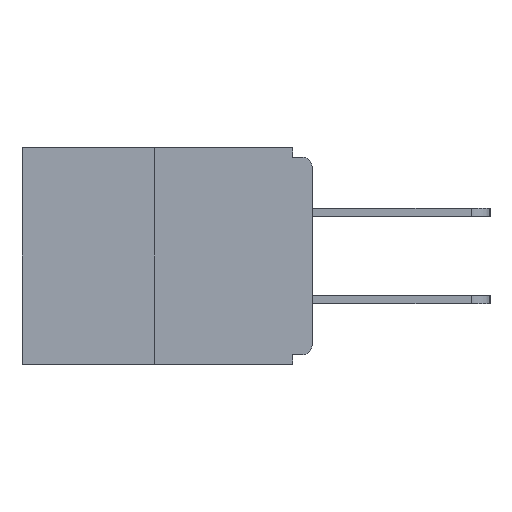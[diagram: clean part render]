
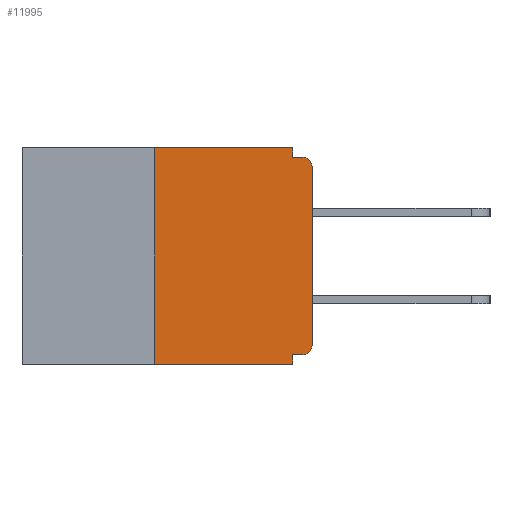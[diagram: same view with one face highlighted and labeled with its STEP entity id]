
A CAD part, left-side view. The second image highlights one B-rep face of the part: STEP entity #11995.
In plain terms, the highlighted planar face has unit normal (-1, 0, 0).
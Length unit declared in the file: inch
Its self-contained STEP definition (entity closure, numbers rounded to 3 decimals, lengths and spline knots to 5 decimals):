
#1243 = CARTESIAN_POINT ( 'NONE',  ( 0., 0.031, 0. ) ) ;
#1306 = CARTESIAN_POINT ( 'NONE',  ( 0., 0.015, -0.313 ) ) ;
#1724 = LINE ( 'NONE', #29578, #30175 ) ;
#1776 = LINE ( 'NONE', #13840, #30394 ) ;
#2646 = AXIS2_PLACEMENT_3D ( 'NONE', #10609, #20037, #5965 ) ;
#2881 = ORIENTED_EDGE ( 'NONE', *, *, #13400, .T. ) ;
#2993 = EDGE_CURVE ( 'NONE', #8689, #3377, #6218, .T. ) ;
#3151 = CIRCLE ( 'NONE', #2646, 0.015 ) ;
#3377 = VERTEX_POINT ( 'NONE', #12689 ) ;
#3730 = LINE ( 'NONE', #1243, #15689 ) ;
#3793 = DIRECTION ( 'NONE',  ( -1., 0., 0. ) ) ;
#4022 = DIRECTION ( 'NONE',  ( 0., 0., -1. ) ) ;
#4214 = VERTEX_POINT ( 'NONE', #24822 ) ;
#4319 = LINE ( 'NONE', #18544, #5563 ) ;
#4607 = VERTEX_POINT ( 'NONE', #19976 ) ;
#5035 = VECTOR ( 'NONE', #22142, 39.37008 ) ;
#5097 = DIRECTION ( 'NONE',  ( 0., 0., 1. ) ) ;
#5397 = VERTEX_POINT ( 'NONE', #9967 ) ;
#5511 = VERTEX_POINT ( 'NONE', #10764 ) ;
#5563 = VECTOR ( 'NONE', #29996, 39.37008 ) ;
#5786 = CARTESIAN_POINT ( 'NONE',  ( 0., 0.46, 0. ) ) ;
#5965 = DIRECTION ( 'NONE',  ( 0., 0., -1. ) ) ;
#5984 = EDGE_CURVE ( 'NONE', #30033, #3377, #1724, .T. ) ;
#6084 = ORIENTED_EDGE ( 'NONE', *, *, #2993, .F. ) ;
#6218 = LINE ( 'NONE', #19815, #5035 ) ;
#6766 = VECTOR ( 'NONE', #22797, 39.37008 ) ;
#6919 = EDGE_CURVE ( 'NONE', #5397, #4214, #12065, .T. ) ;
#7158 = FACE_OUTER_BOUND ( 'NONE', #22399, .T. ) ;
#8475 = CARTESIAN_POINT ( 'NONE',  ( 0., 0.25, 0. ) ) ;
#8637 = ORIENTED_EDGE ( 'NONE', *, *, #16907, .F. ) ;
#8689 = VERTEX_POINT ( 'NONE', #18359 ) ;
#9343 = DIRECTION ( 'NONE',  ( 0., -1., 0. ) ) ;
#9407 = VECTOR ( 'NONE', #5097, 39.37008 ) ;
#9967 = CARTESIAN_POINT ( 'NONE',  ( 0., 0., -0.313 ) ) ;
#10609 = CARTESIAN_POINT ( 'NONE',  ( 0., 0.015, -0.03 ) ) ;
#10764 = CARTESIAN_POINT ( 'NONE',  ( 0., 0.015, -0.015 ) ) ;
#11325 = DIRECTION ( 'NONE',  ( 0., -1., 0. ) ) ;
#11995 = ADVANCED_FACE ( 'NONE', ( #7158 ), #15229, .F. ) ;
#12065 = LINE ( 'NONE', #21492, #9407 ) ;
#12082 = CARTESIAN_POINT ( 'NONE',  ( 0., 0., -0.015 ) ) ;
#12445 = ORIENTED_EDGE ( 'NONE', *, *, #5984, .T. ) ;
#12496 = AXIS2_PLACEMENT_3D ( 'NONE', #1306, #3793, #13376 ) ;
#12531 = EDGE_CURVE ( 'NONE', #19937, #8689, #4319, .T. ) ;
#12689 = CARTESIAN_POINT ( 'NONE',  ( 0., 0.031, -0.343 ) ) ;
#13239 = ORIENTED_EDGE ( 'NONE', *, *, #6919, .T. ) ;
#13291 = LINE ( 'NONE', #8475, #24461 ) ;
#13376 = DIRECTION ( 'NONE',  ( 0., 0., -1. ) ) ;
#13400 = EDGE_CURVE ( 'NONE', #19937, #5397, #25824, .T. ) ;
#13840 = CARTESIAN_POINT ( 'NONE',  ( 0., 0.46, 0. ) ) ;
#13953 = ORIENTED_EDGE ( 'NONE', *, *, #27758, .F. ) ;
#14641 = CARTESIAN_POINT ( 'NONE',  ( 0., 0.031, 0. ) ) ;
#15158 = ORIENTED_EDGE ( 'NONE', *, *, #23661, .F. ) ;
#15229 = PLANE ( 'NONE',  #29943 ) ;
#15689 = VECTOR ( 'NONE', #4022, 39.37008 ) ;
#16850 = CARTESIAN_POINT ( 'NONE',  ( 0., 0.25, -0.343 ) ) ;
#16907 = EDGE_CURVE ( 'NONE', #30033, #27352, #13291, .T. ) ;
#18359 = CARTESIAN_POINT ( 'NONE',  ( 0., 0.031, -0.328 ) ) ;
#18369 = CARTESIAN_POINT ( 'NONE',  ( 0., 0.25, 0. ) ) ;
#18544 = CARTESIAN_POINT ( 'NONE',  ( 0., 0., -0.328 ) ) ;
#19815 = CARTESIAN_POINT ( 'NONE',  ( 0., 0.031, -0.343 ) ) ;
#19937 = VERTEX_POINT ( 'NONE', #26361 ) ;
#19976 = CARTESIAN_POINT ( 'NONE',  ( 0., 0.031, -0.015 ) ) ;
#20037 = DIRECTION ( 'NONE',  ( -1., 0., 0. ) ) ;
#20489 = LINE ( 'NONE', #12082, #6766 ) ;
#21492 = CARTESIAN_POINT ( 'NONE',  ( 0., 0., 0. ) ) ;
#22010 = DIRECTION ( 'NONE',  ( 0., 0., -1. ) ) ;
#22142 = DIRECTION ( 'NONE',  ( 0., 0., -1. ) ) ;
#22399 = EDGE_LOOP ( 'NONE', ( #13953, #8637, #12445, #6084, #23421, #2881, #13239, #24685, #15158, #28193 ) ) ;
#22797 = DIRECTION ( 'NONE',  ( 0., -1., 0. ) ) ;
#23421 = ORIENTED_EDGE ( 'NONE', *, *, #12531, .F. ) ;
#23661 = EDGE_CURVE ( 'NONE', #4607, #5511, #20489, .T. ) ;
#23829 = EDGE_CURVE ( 'NONE', #28844, #4607, #3730, .T. ) ;
#24461 = VECTOR ( 'NONE', #24889, 39.37008 ) ;
#24685 = ORIENTED_EDGE ( 'NONE', *, *, #24843, .T. ) ;
#24822 = CARTESIAN_POINT ( 'NONE',  ( 0., 0., -0.03 ) ) ;
#24843 = EDGE_CURVE ( 'NONE', #4214, #5511, #3151, .T. ) ;
#24889 = DIRECTION ( 'NONE',  ( 0., 0., 1. ) ) ;
#25824 = CIRCLE ( 'NONE', #12496, 0.015 ) ;
#26361 = CARTESIAN_POINT ( 'NONE',  ( 0., 0.015, -0.328 ) ) ;
#27352 = VERTEX_POINT ( 'NONE', #18369 ) ;
#27758 = EDGE_CURVE ( 'NONE', #27352, #28844, #1776, .T. ) ;
#28193 = ORIENTED_EDGE ( 'NONE', *, *, #23829, .F. ) ;
#28844 = VERTEX_POINT ( 'NONE', #14641 ) ;
#29118 = DIRECTION ( 'NONE',  ( 1., 0., 0. ) ) ;
#29578 = CARTESIAN_POINT ( 'NONE',  ( 0., 0.46, -0.343 ) ) ;
#29943 = AXIS2_PLACEMENT_3D ( 'NONE', #5786, #29118, #22010 ) ;
#29996 = DIRECTION ( 'NONE',  ( 0., 1., 0. ) ) ;
#30033 = VERTEX_POINT ( 'NONE', #16850 ) ;
#30175 = VECTOR ( 'NONE', #11325, 39.37008 ) ;
#30394 = VECTOR ( 'NONE', #9343, 39.37008 ) ;
